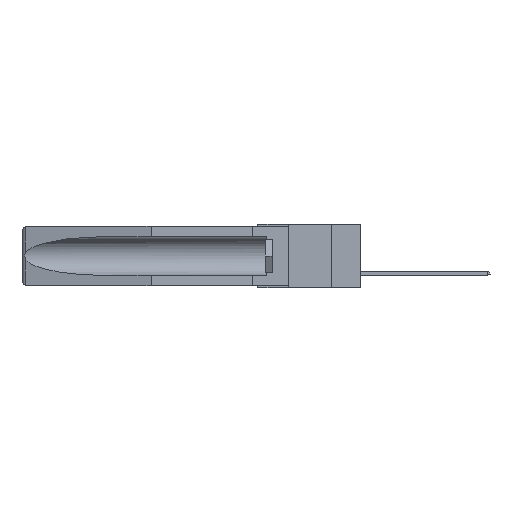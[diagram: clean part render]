
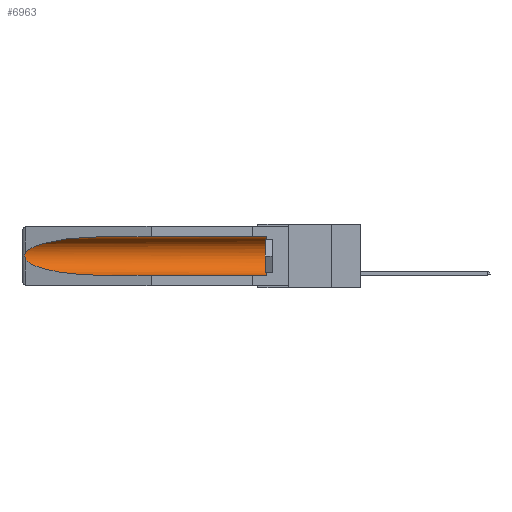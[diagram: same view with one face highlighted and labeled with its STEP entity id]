
A CAD part, left-side view. The second image highlights one B-rep face of the part: STEP entity #6963.
In plain terms, the highlighted cylindrical face has radius 2.857 mm (diameter 5.715 mm), a partial arc.
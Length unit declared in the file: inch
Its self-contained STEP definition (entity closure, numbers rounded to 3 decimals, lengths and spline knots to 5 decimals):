
#878 = EDGE_CURVE ( 'NONE', #15605, #21937, #7842, .T. ) ;
#1290 = DIRECTION ( 'NONE',  ( 0., 0., 1. ) ) ;
#1912 = EDGE_CURVE ( 'NONE', #18146, #10813, #10245, .T. ) ;
#2346 = DIRECTION ( 'NONE',  ( 0., 1., 0. ) ) ;
#2545 =( BOUNDED_CURVE ( )  B_SPLINE_CURVE ( 3, ( #15447, #6822, #21259, #25468 ),
 .UNSPECIFIED., .F., .F. ) 
 B_SPLINE_CURVE_WITH_KNOTS ( ( 4, 4 ),
 ( 4.71239, 6.08839 ),
 .UNSPECIFIED. ) 
 CURVE ( )  GEOMETRIC_REPRESENTATION_ITEM ( )  RATIONAL_B_SPLINE_CURVE ( ( 1., 0.848, 0.848, 1. ) ) 
 REPRESENTATION_ITEM ( '' )  );
#2571 = DIRECTION ( 'NONE',  ( 0., 1., 0. ) ) ;
#2593 = VERTEX_POINT ( 'NONE', #19024 ) ;
#3168 = CARTESIAN_POINT ( 'NONE',  ( 0.26655, 1.53094, -0.18657 ) ) ;
#4018 = CARTESIAN_POINT ( 'NONE',  ( 0.21114, 1.30732, -0.284 ) ) ;
#4721 = EDGE_CURVE ( 'NONE', #26515, #2593, #19495, .T. ) ;
#4962 = CARTESIAN_POINT ( 'NONE',  ( 0.155, -0.30754, -0.1715 ) ) ;
#5282 = VECTOR ( 'NONE', #18325, 39.37008 ) ;
#5983 = CARTESIAN_POINT ( 'NONE',  ( 0.155, 1.07973, -0.284 ) ) ;
#6822 = CARTESIAN_POINT ( 'NONE',  ( 0.21114, 1.30732, -0.059 ) ) ;
#6963 = ADVANCED_FACE ( 'NONE', ( #7359 ), #26461, .F. ) ;
#7359 = FACE_OUTER_BOUND ( 'NONE', #19994, .T. ) ;
#7469 = CARTESIAN_POINT ( 'NONE',  ( 0.2673, 1.53269, -0.17917 ) ) ;
#7730 = CARTESIAN_POINT ( 'NONE',  ( 0.26537, 1.52718, -0.19328 ) ) ;
#7842 = LINE ( 'NONE', #20036, #5282 ) ;
#9552 = CARTESIAN_POINT ( 'NONE',  ( 0.26597, 1.5296, -0.19026 ) ) ;
#10245 = B_SPLINE_CURVE_WITH_KNOTS ( 'NONE', 3,
 ( #23823, #11448, #25928, #15722, #19821, #24003, #7469, #3168, #9552, #13737 ),
 .UNSPECIFIED., .F., .F.,
 ( 4, 2, 2, 2, 4 ),
 ( 0., 0.00029, 0.00058, 0.00087, 0.00117 ),
 .UNSPECIFIED. ) ;
#10813 = VERTEX_POINT ( 'NONE', #7730 ) ;
#10934 = DIRECTION ( 'NONE',  ( 0., 0., 1. ) ) ;
#11060 = EDGE_CURVE ( 'NONE', #10813, #21937, #13434, .T. ) ;
#11448 = CARTESIAN_POINT ( 'NONE',  ( 0.26597, 1.52961, -0.15275 ) ) ;
#11739 = DIRECTION ( 'NONE',  ( 0., -1., 0. ) ) ;
#11874 = ORIENTED_EDGE ( 'NONE', *, *, #4721, .T. ) ;
#12080 = CIRCLE ( 'NONE', #14167, 0.1125 ) ;
#12582 = CARTESIAN_POINT ( 'NONE',  ( 0.155, 1.07973, -0.284 ) ) ;
#12877 = ORIENTED_EDGE ( 'NONE', *, *, #1912, .T. ) ;
#13434 =( BOUNDED_CURVE ( )  B_SPLINE_CURVE ( 3, ( #16455, #16655, #4018, #12582 ),
 .UNSPECIFIED., .F., .F. ) 
 B_SPLINE_CURVE_WITH_KNOTS ( ( 4, 4 ),
 ( 0.1948, 1.5708 ),
 .UNSPECIFIED. ) 
 CURVE ( )  GEOMETRIC_REPRESENTATION_ITEM ( )  RATIONAL_B_SPLINE_CURVE ( ( 1., 0.848, 0.848, 1. ) ) 
 REPRESENTATION_ITEM ( '' )  );
#13737 = CARTESIAN_POINT ( 'NONE',  ( 0.26537, 1.52718, -0.19328 ) ) ;
#14167 = AXIS2_PLACEMENT_3D ( 'NONE', #24127, #11739, #1290 ) ;
#15173 = CARTESIAN_POINT ( 'NONE',  ( 0.155, 0.126, -0.284 ) ) ;
#15447 = CARTESIAN_POINT ( 'NONE',  ( 0.155, 1.07973, -0.059 ) ) ;
#15605 = VERTEX_POINT ( 'NONE', #15173 ) ;
#15722 = CARTESIAN_POINT ( 'NONE',  ( 0.2673, 1.5327, -0.16383 ) ) ;
#16455 = CARTESIAN_POINT ( 'NONE',  ( 0.26537, 1.52718, -0.19328 ) ) ;
#16655 = CARTESIAN_POINT ( 'NONE',  ( 0.25451, 1.48313, -0.24835 ) ) ;
#18146 = VERTEX_POINT ( 'NONE', #24632 ) ;
#18325 = DIRECTION ( 'NONE',  ( 0., 1., 0. ) ) ;
#18628 = EDGE_CURVE ( 'NONE', #15605, #26515, #12080, .T. ) ;
#19024 = CARTESIAN_POINT ( 'NONE',  ( 0.155, 1.07973, -0.059 ) ) ;
#19495 = LINE ( 'NONE', #24998, #21418 ) ;
#19821 = CARTESIAN_POINT ( 'NONE',  ( 0.2675, 1.53308, -0.16763 ) ) ;
#19994 = EDGE_LOOP ( 'NONE', ( #25838, #12877, #22703, #24370, #23605, #11874 ) ) ;
#20036 = CARTESIAN_POINT ( 'NONE',  ( 0.155, -0.30754, -0.284 ) ) ;
#20980 = EDGE_CURVE ( 'NONE', #2593, #18146, #2545, .T. ) ;
#21259 = CARTESIAN_POINT ( 'NONE',  ( 0.25451, 1.48313, -0.09465 ) ) ;
#21418 = VECTOR ( 'NONE', #2346, 39.37008 ) ;
#21937 = VERTEX_POINT ( 'NONE', #5983 ) ;
#22407 = CARTESIAN_POINT ( 'NONE',  ( 0.155, 0.126, -0.059 ) ) ;
#22703 = ORIENTED_EDGE ( 'NONE', *, *, #11060, .T. ) ;
#23435 = AXIS2_PLACEMENT_3D ( 'NONE', #4962, #2571, #10934 ) ;
#23605 = ORIENTED_EDGE ( 'NONE', *, *, #18628, .T. ) ;
#23823 = CARTESIAN_POINT ( 'NONE',  ( 0.26537, 1.52718, -0.14972 ) ) ;
#24003 = CARTESIAN_POINT ( 'NONE',  ( 0.2675, 1.53308, -0.17534 ) ) ;
#24127 = CARTESIAN_POINT ( 'NONE',  ( 0.155, 0.126, -0.1715 ) ) ;
#24370 = ORIENTED_EDGE ( 'NONE', *, *, #878, .F. ) ;
#24632 = CARTESIAN_POINT ( 'NONE',  ( 0.26537, 1.52718, -0.14972 ) ) ;
#24998 = CARTESIAN_POINT ( 'NONE',  ( 0.155, -0.30754, -0.059 ) ) ;
#25468 = CARTESIAN_POINT ( 'NONE',  ( 0.26537, 1.52718, -0.14972 ) ) ;
#25838 = ORIENTED_EDGE ( 'NONE', *, *, #20980, .T. ) ;
#25928 = CARTESIAN_POINT ( 'NONE',  ( 0.26654, 1.53092, -0.15636 ) ) ;
#26461 = CYLINDRICAL_SURFACE ( 'NONE', #23435, 0.1125 ) ;
#26515 = VERTEX_POINT ( 'NONE', #22407 ) ;
